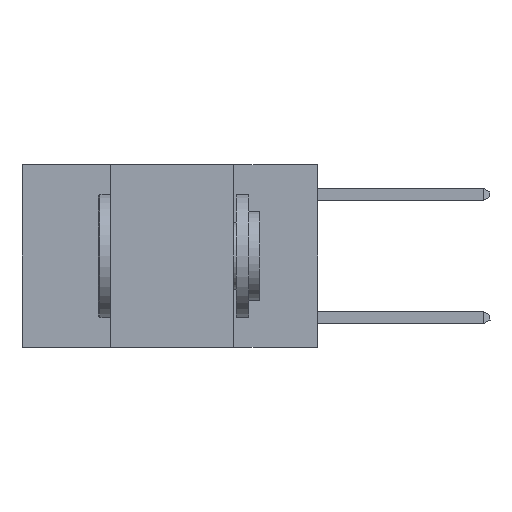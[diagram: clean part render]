
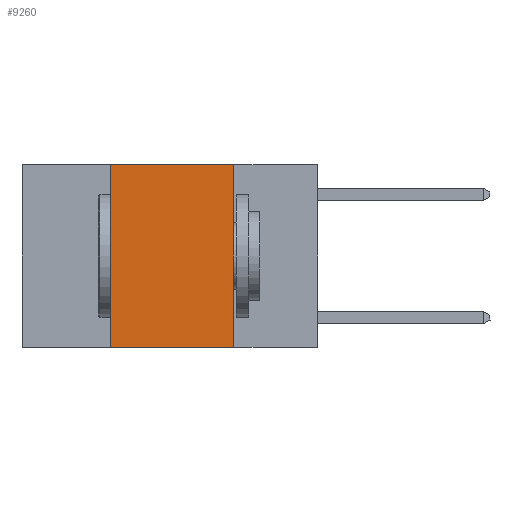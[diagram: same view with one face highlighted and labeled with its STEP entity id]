
A CAD part, left-side view. The second image highlights one B-rep face of the part: STEP entity #9260.
In plain terms, the highlighted planar face has unit normal (-1, 0, 0).
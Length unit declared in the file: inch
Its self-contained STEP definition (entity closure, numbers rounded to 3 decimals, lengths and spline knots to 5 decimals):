
#1465 = VECTOR ( 'NONE', #18410, 39.37008 ) ;
#1802 = EDGE_CURVE ( 'NONE', #9222, #20393, #11543, .T. ) ;
#3307 = CARTESIAN_POINT ( 'NONE',  ( 0., 0.17, -0.37 ) ) ;
#3352 = CARTESIAN_POINT ( 'NONE',  ( 0., 0.42, -0.37 ) ) ;
#3442 = CARTESIAN_POINT ( 'NONE',  ( 0., 0.6, 0. ) ) ;
#3703 = VERTEX_POINT ( 'NONE', #18602 ) ;
#3962 = DIRECTION ( 'NONE',  ( 0., -1., 0. ) ) ;
#4396 = ORIENTED_EDGE ( 'NONE', *, *, #7351, .F. ) ;
#5841 = DIRECTION ( 'NONE',  ( 0., 0., -1. ) ) ;
#5863 = VECTOR ( 'NONE', #3962, 39.37008 ) ;
#7351 = EDGE_CURVE ( 'NONE', #9222, #8066, #18326, .T. ) ;
#7831 = DIRECTION ( 'NONE',  ( 0., 0., -1. ) ) ;
#7913 = DIRECTION ( 'NONE',  ( 0., 0., 1. ) ) ;
#8066 = VERTEX_POINT ( 'NONE', #25013 ) ;
#9222 = VERTEX_POINT ( 'NONE', #3352 ) ;
#9260 = ADVANCED_FACE ( 'NONE', ( #27445 ), #14195, .F. ) ;
#11063 = ORIENTED_EDGE ( 'NONE', *, *, #21788, .F. ) ;
#11543 = LINE ( 'NONE', #18878, #5863 ) ;
#12312 = CARTESIAN_POINT ( 'NONE',  ( 0., 0.17, 0. ) ) ;
#14114 = CARTESIAN_POINT ( 'NONE',  ( 0., 0.6, 0. ) ) ;
#14177 = VECTOR ( 'NONE', #5841, 39.37008 ) ;
#14195 = PLANE ( 'NONE',  #21756 ) ;
#14334 = EDGE_LOOP ( 'NONE', ( #11063, #17463, #4396, #25808 ) ) ;
#14390 = CARTESIAN_POINT ( 'NONE',  ( 0., 0.42, 0. ) ) ;
#17463 = ORIENTED_EDGE ( 'NONE', *, *, #19148, .F. ) ;
#17683 = VECTOR ( 'NONE', #7913, 39.37008 ) ;
#18005 = LINE ( 'NONE', #14114, #1465 ) ;
#18326 = LINE ( 'NONE', #14390, #17683 ) ;
#18410 = DIRECTION ( 'NONE',  ( 0., -1., 0. ) ) ;
#18602 = CARTESIAN_POINT ( 'NONE',  ( 0., 0.17, 0. ) ) ;
#18878 = CARTESIAN_POINT ( 'NONE',  ( 0., 0.6, -0.37 ) ) ;
#19148 = EDGE_CURVE ( 'NONE', #8066, #3703, #18005, .T. ) ;
#19176 = LINE ( 'NONE', #12312, #14177 ) ;
#20393 = VERTEX_POINT ( 'NONE', #3307 ) ;
#20583 = DIRECTION ( 'NONE',  ( 1., 0., 0. ) ) ;
#21756 = AXIS2_PLACEMENT_3D ( 'NONE', #3442, #20583, #7831 ) ;
#21788 = EDGE_CURVE ( 'NONE', #3703, #20393, #19176, .T. ) ;
#25013 = CARTESIAN_POINT ( 'NONE',  ( 0., 0.42, 0. ) ) ;
#25808 = ORIENTED_EDGE ( 'NONE', *, *, #1802, .T. ) ;
#27445 = FACE_OUTER_BOUND ( 'NONE', #14334, .T. ) ;
